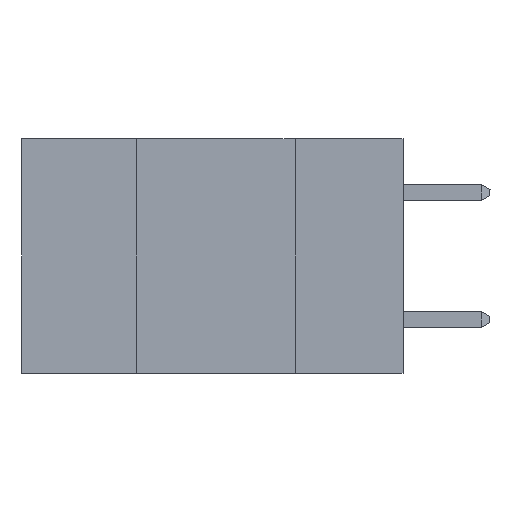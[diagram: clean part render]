
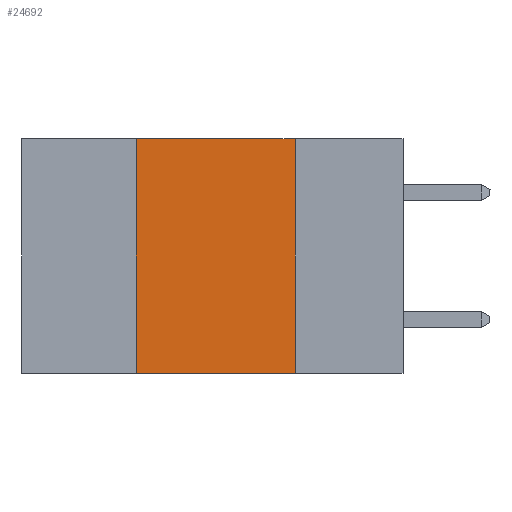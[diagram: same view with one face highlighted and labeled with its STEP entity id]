
A CAD part, left-side view. The second image highlights one B-rep face of the part: STEP entity #24692.
In plain terms, the highlighted planar face has unit normal (-1, 0, 0).
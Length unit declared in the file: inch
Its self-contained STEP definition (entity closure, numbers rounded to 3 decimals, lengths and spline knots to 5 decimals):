
#30 = DIRECTION ( 'NONE',  ( 0., -1., 0. ) ) ;
#1215 = ORIENTED_EDGE ( 'NONE', *, *, #3604, .T. ) ;
#1581 = EDGE_CURVE ( 'NONE', #6081, #3042, #5046, .T. ) ;
#3042 = VERTEX_POINT ( 'NONE', #7802 ) ;
#3152 = CARTESIAN_POINT ( 'NONE',  ( 0., 0.6, 0. ) ) ;
#3604 = EDGE_CURVE ( 'NONE', #24266, #5852, #7446, .T. ) ;
#5046 = LINE ( 'NONE', #16521, #29795 ) ;
#5075 = DIRECTION ( 'NONE',  ( 0., -1., 0. ) ) ;
#5852 = VERTEX_POINT ( 'NONE', #24583 ) ;
#6081 = VERTEX_POINT ( 'NONE', #20947 ) ;
#7356 = VECTOR ( 'NONE', #5075, 39.37008 ) ;
#7446 = LINE ( 'NONE', #16849, #7356 ) ;
#7565 = FACE_OUTER_BOUND ( 'NONE', #11269, .T. ) ;
#7802 = CARTESIAN_POINT ( 'NONE',  ( 0., 0.17, 0. ) ) ;
#8800 = CARTESIAN_POINT ( 'NONE',  ( 0., 0.42, 0. ) ) ;
#10058 = AXIS2_PLACEMENT_3D ( 'NONE', #3152, #10059, #24616 ) ;
#10059 = DIRECTION ( 'NONE',  ( 1., 0., 0. ) ) ;
#11269 = EDGE_LOOP ( 'NONE', ( #24876, #21121, #24414, #1215 ) ) ;
#11447 = DIRECTION ( 'NONE',  ( 0., 0., 1. ) ) ;
#12339 = CARTESIAN_POINT ( 'NONE',  ( 0., 0.42, -0.37 ) ) ;
#15992 = LINE ( 'NONE', #25517, #24712 ) ;
#16010 = LINE ( 'NONE', #8800, #23428 ) ;
#16521 = CARTESIAN_POINT ( 'NONE',  ( 0., 0.6, 0. ) ) ;
#16849 = CARTESIAN_POINT ( 'NONE',  ( 0., 0.6, -0.37 ) ) ;
#19492 = EDGE_CURVE ( 'NONE', #24266, #6081, #16010, .T. ) ;
#20947 = CARTESIAN_POINT ( 'NONE',  ( 0., 0.42, 0. ) ) ;
#21121 = ORIENTED_EDGE ( 'NONE', *, *, #1581, .F. ) ;
#21962 = PLANE ( 'NONE',  #10058 ) ;
#23428 = VECTOR ( 'NONE', #11447, 39.37008 ) ;
#24266 = VERTEX_POINT ( 'NONE', #12339 ) ;
#24414 = ORIENTED_EDGE ( 'NONE', *, *, #19492, .F. ) ;
#24583 = CARTESIAN_POINT ( 'NONE',  ( 0., 0.17, -0.37 ) ) ;
#24616 = DIRECTION ( 'NONE',  ( 0., 0., -1. ) ) ;
#24692 = ADVANCED_FACE ( 'NONE', ( #7565 ), #21962, .F. ) ;
#24712 = VECTOR ( 'NONE', #28776, 39.37008 ) ;
#24876 = ORIENTED_EDGE ( 'NONE', *, *, #26749, .F. ) ;
#25517 = CARTESIAN_POINT ( 'NONE',  ( 0., 0.17, 0. ) ) ;
#26749 = EDGE_CURVE ( 'NONE', #3042, #5852, #15992, .T. ) ;
#28776 = DIRECTION ( 'NONE',  ( 0., 0., -1. ) ) ;
#29795 = VECTOR ( 'NONE', #30, 39.37008 ) ;
